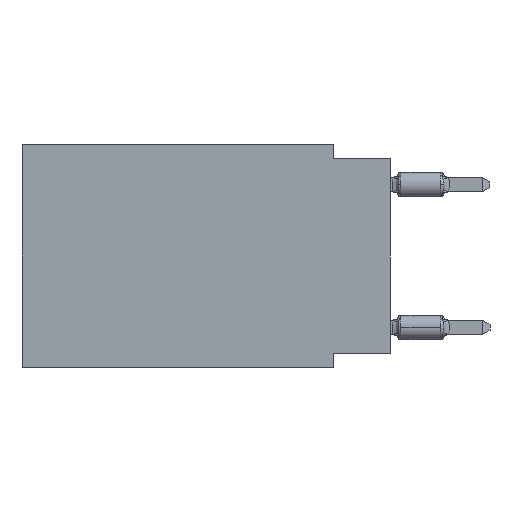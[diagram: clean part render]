
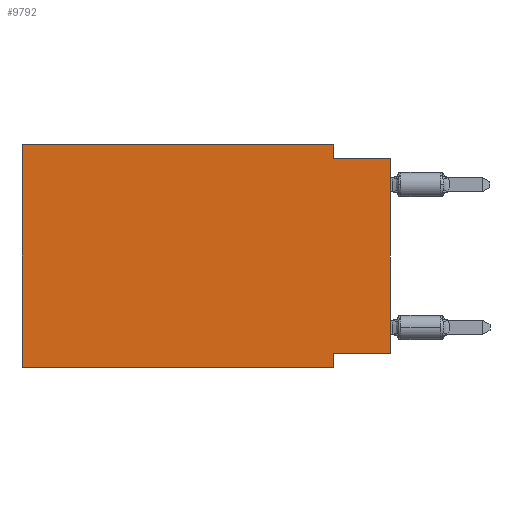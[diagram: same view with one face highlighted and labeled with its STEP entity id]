
A CAD part, left-side view. The second image highlights one B-rep face of the part: STEP entity #9792.
In plain terms, the highlighted planar face has unit normal (-1, 0, 0).
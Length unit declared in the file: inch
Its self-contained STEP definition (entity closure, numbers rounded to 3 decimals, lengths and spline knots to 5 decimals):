
#12 = EDGE_CURVE ( 'NONE', #21378, #3943, #19684, .T. ) ;
#577 = DIRECTION ( 'NONE',  ( 0., 1., 0. ) ) ;
#946 = VECTOR ( 'NONE', #577, 39.37008 ) ;
#2501 = VERTEX_POINT ( 'NONE', #30362 ) ;
#2630 = EDGE_CURVE ( 'NONE', #12541, #33381, #23419, .T. ) ;
#3605 = FACE_OUTER_BOUND ( 'NONE', #35361, .T. ) ;
#3922 = VECTOR ( 'NONE', #35839, 39.37008 ) ;
#3943 = VERTEX_POINT ( 'NONE', #33193 ) ;
#4581 = CARTESIAN_POINT ( 'NONE',  ( 0., 0., -0.025 ) ) ;
#5005 = VERTEX_POINT ( 'NONE', #6073 ) ;
#5043 = CARTESIAN_POINT ( 'NONE',  ( 0., 0.645, 0. ) ) ;
#5236 = ORIENTED_EDGE ( 'NONE', *, *, #5322, .T. ) ;
#5322 = EDGE_CURVE ( 'NONE', #6220, #5005, #11538, .T. ) ;
#5694 = DIRECTION ( 'NONE',  ( 0., -1., 0. ) ) ;
#6029 = ORIENTED_EDGE ( 'NONE', *, *, #7141, .T. ) ;
#6073 = CARTESIAN_POINT ( 'NONE',  ( 0., 0.1, -0.39 ) ) ;
#6076 = CARTESIAN_POINT ( 'NONE',  ( 0., 0.1, 0. ) ) ;
#6220 = VERTEX_POINT ( 'NONE', #32984 ) ;
#7141 = EDGE_CURVE ( 'NONE', #21378, #28140, #31996, .T. ) ;
#7224 = ORIENTED_EDGE ( 'NONE', *, *, #26218, .F. ) ;
#7581 = EDGE_CURVE ( 'NONE', #2501, #28140, #29313, .T. ) ;
#7769 = CARTESIAN_POINT ( 'NONE',  ( 0., 0., -0.025 ) ) ;
#8169 = ORIENTED_EDGE ( 'NONE', *, *, #26827, .F. ) ;
#9792 = ADVANCED_FACE ( 'NONE', ( #3605 ), #19086, .F. ) ;
#10945 = DIRECTION ( 'NONE',  ( 0., -1., 0. ) ) ;
#11538 = LINE ( 'NONE', #30458, #12296 ) ;
#12296 = VECTOR ( 'NONE', #5694, 39.37008 ) ;
#12541 = VERTEX_POINT ( 'NONE', #5043 ) ;
#14296 = CARTESIAN_POINT ( 'NONE',  ( 0., 0., -0.365 ) ) ;
#14374 = CARTESIAN_POINT ( 'NONE',  ( 0., 0.645, 0. ) ) ;
#14933 = ORIENTED_EDGE ( 'NONE', *, *, #12, .F. ) ;
#17335 = LINE ( 'NONE', #29611, #3922 ) ;
#18671 = LINE ( 'NONE', #19258, #27417 ) ;
#19086 = PLANE ( 'NONE',  #22876 ) ;
#19258 = CARTESIAN_POINT ( 'NONE',  ( 0., 0.645, 0. ) ) ;
#19611 = LINE ( 'NONE', #31889, #30671 ) ;
#19684 = LINE ( 'NONE', #37417, #946 ) ;
#20010 = EDGE_CURVE ( 'NONE', #33381, #2501, #19611, .T. ) ;
#21378 = VERTEX_POINT ( 'NONE', #14296 ) ;
#21931 = CARTESIAN_POINT ( 'NONE',  ( 0., 0.645, 0. ) ) ;
#22876 = AXIS2_PLACEMENT_3D ( 'NONE', #21931, #24907, #37205 ) ;
#23365 = VECTOR ( 'NONE', #26338, 39.37008 ) ;
#23419 = LINE ( 'NONE', #14374, #30873 ) ;
#24907 = DIRECTION ( 'NONE',  ( 1., 0., 0. ) ) ;
#25089 = DIRECTION ( 'NONE',  ( 0., 0., 1. ) ) ;
#26098 = DIRECTION ( 'NONE',  ( 0., -1., 0. ) ) ;
#26218 = EDGE_CURVE ( 'NONE', #3943, #5005, #17335, .T. ) ;
#26338 = DIRECTION ( 'NONE',  ( 0., 0., 1. ) ) ;
#26827 = EDGE_CURVE ( 'NONE', #6220, #12541, #18671, .T. ) ;
#27109 = ORIENTED_EDGE ( 'NONE', *, *, #7581, .F. ) ;
#27417 = VECTOR ( 'NONE', #25089, 39.37008 ) ;
#28140 = VERTEX_POINT ( 'NONE', #4581 ) ;
#29256 = DIRECTION ( 'NONE',  ( 0., 0., -1. ) ) ;
#29313 = LINE ( 'NONE', #7769, #36906 ) ;
#29611 = CARTESIAN_POINT ( 'NONE',  ( 0., 0.1, -0.39 ) ) ;
#30362 = CARTESIAN_POINT ( 'NONE',  ( 0., 0.1, -0.025 ) ) ;
#30458 = CARTESIAN_POINT ( 'NONE',  ( 0., 0.645, -0.39 ) ) ;
#30671 = VECTOR ( 'NONE', #29256, 39.37008 ) ;
#30873 = VECTOR ( 'NONE', #10945, 39.37008 ) ;
#31320 = ORIENTED_EDGE ( 'NONE', *, *, #20010, .F. ) ;
#31794 = CARTESIAN_POINT ( 'NONE',  ( 0., 0., 0. ) ) ;
#31889 = CARTESIAN_POINT ( 'NONE',  ( 0., 0.1, 0. ) ) ;
#31996 = LINE ( 'NONE', #31794, #23365 ) ;
#32984 = CARTESIAN_POINT ( 'NONE',  ( 0., 0.645, -0.39 ) ) ;
#33193 = CARTESIAN_POINT ( 'NONE',  ( 0., 0.1, -0.365 ) ) ;
#33381 = VERTEX_POINT ( 'NONE', #6076 ) ;
#35361 = EDGE_LOOP ( 'NONE', ( #6029, #27109, #31320, #36686, #8169, #5236, #7224, #14933 ) ) ;
#35839 = DIRECTION ( 'NONE',  ( 0., 0., -1. ) ) ;
#36686 = ORIENTED_EDGE ( 'NONE', *, *, #2630, .F. ) ;
#36906 = VECTOR ( 'NONE', #26098, 39.37008 ) ;
#37205 = DIRECTION ( 'NONE',  ( 0., 0., -1. ) ) ;
#37417 = CARTESIAN_POINT ( 'NONE',  ( 0., 0., -0.365 ) ) ;
